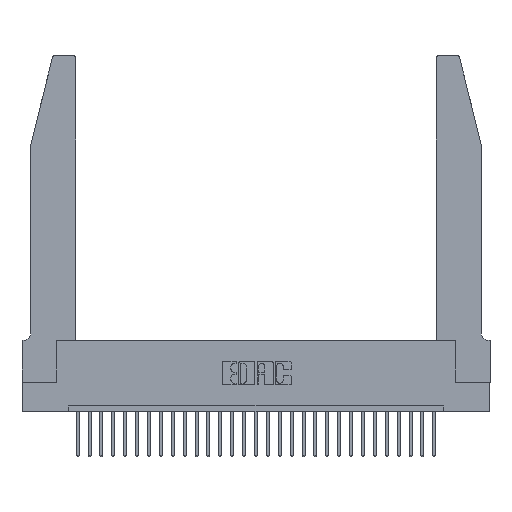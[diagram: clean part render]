
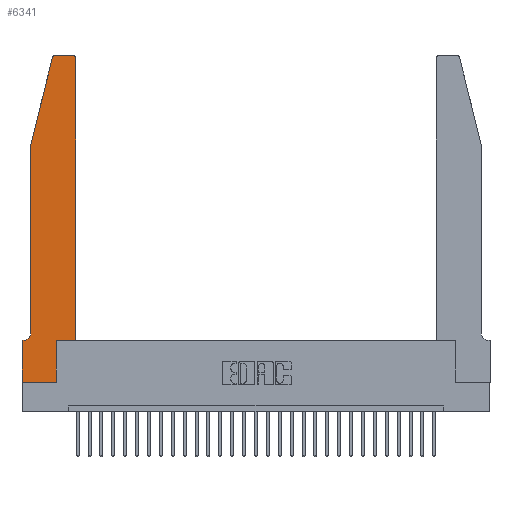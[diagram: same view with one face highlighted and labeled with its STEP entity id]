
A CAD part, top view. The second image highlights one B-rep face of the part: STEP entity #6341.
In plain terms, the highlighted planar face has unit normal (0, 0, 1).
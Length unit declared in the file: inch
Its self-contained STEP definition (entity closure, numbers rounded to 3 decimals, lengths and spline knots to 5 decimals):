
#595 = ORIENTED_EDGE ( 'NONE', *, *, #10351, .T. ) ;
#735 = ORIENTED_EDGE ( 'NONE', *, *, #6248, .T. ) ;
#934 = CARTESIAN_POINT ( 'NONE',  ( 0.0755, 0.35, 0.37 ) ) ;
#1357 = CARTESIAN_POINT ( 'NONE',  ( 0.25487, 2.72718, 0.37 ) ) ;
#1361 = ORIENTED_EDGE ( 'NONE', *, *, #3105, .T. ) ;
#1368 = EDGE_CURVE ( 'NONE', #23495, #5589, #11917, .T. ) ;
#1647 = CARTESIAN_POINT ( 'NONE',  ( 0., 0., 0.37 ) ) ;
#1917 = CARTESIAN_POINT ( 'NONE',  ( 0., 0., 0.37 ) ) ;
#2184 = ORIENTED_EDGE ( 'NONE', *, *, #26930, .T. ) ;
#2777 = CARTESIAN_POINT ( 'NONE',  ( 0.284, 2.72, 0.37 ) ) ;
#3105 = EDGE_CURVE ( 'NONE', #5589, #27038, #28987, .T. ) ;
#3804 = ORIENTED_EDGE ( 'NONE', *, *, #10333, .T. ) ;
#4568 = LINE ( 'NONE', #23553, #22810 ) ;
#4655 = CARTESIAN_POINT ( 'NONE',  ( 0.4505, 2.72, 0.37 ) ) ;
#4871 = VECTOR ( 'NONE', #26889, 39.37008 ) ;
#5257 = DIRECTION ( 'NONE',  ( 1., 0., 0. ) ) ;
#5456 = VERTEX_POINT ( 'NONE', #12390 ) ;
#5538 = DIRECTION ( 'NONE',  ( 0., 0., 1. ) ) ;
#5582 = CARTESIAN_POINT ( 'NONE',  ( 0.4505, 0.35, 0.37 ) ) ;
#5589 = VERTEX_POINT ( 'NONE', #27062 ) ;
#5603 = CIRCLE ( 'NONE', #28154, 0.07 ) ;
#5796 = LINE ( 'NONE', #25806, #15432 ) ;
#5948 = EDGE_CURVE ( 'NONE', #5456, #9611, #22768, .T. ) ;
#6243 = VERTEX_POINT ( 'NONE', #16514 ) ;
#6248 = EDGE_CURVE ( 'NONE', #14806, #23495, #5603, .T. ) ;
#6341 = ADVANCED_FACE ( 'NONE', ( #29182 ), #28057, .T. ) ;
#6641 = LINE ( 'NONE', #22114, #19127 ) ;
#7485 = ORIENTED_EDGE ( 'NONE', *, *, #12717, .T. ) ;
#7992 = CIRCLE ( 'NONE', #11518, 0.03 ) ;
#9493 = LINE ( 'NONE', #1917, #4871 ) ;
#9611 = VERTEX_POINT ( 'NONE', #21404 ) ;
#9861 = VECTOR ( 'NONE', #11960, 39.37008 ) ;
#9874 = ORIENTED_EDGE ( 'NONE', *, *, #5948, .T. ) ;
#10333 = EDGE_CURVE ( 'NONE', #9611, #28482, #19593, .T. ) ;
#10351 = EDGE_CURVE ( 'NONE', #28482, #28876, #4568, .T. ) ;
#10676 = DIRECTION ( 'NONE',  ( 0., -1., 0. ) ) ;
#11081 = CARTESIAN_POINT ( 'NONE',  ( 0.2865, 0., 0.37 ) ) ;
#11518 = AXIS2_PLACEMENT_3D ( 'NONE', #19491, #15108, #14905 ) ;
#11917 = LINE ( 'NONE', #934, #17292 ) ;
#11960 = DIRECTION ( 'NONE',  ( -1., 0., 0. ) ) ;
#12302 = CARTESIAN_POINT ( 'NONE',  ( 0.0055, 0.42, 0.37 ) ) ;
#12317 = VERTEX_POINT ( 'NONE', #5582 ) ;
#12390 = CARTESIAN_POINT ( 'NONE',  ( 0.4205, 2.75, 0.37 ) ) ;
#12717 = EDGE_CURVE ( 'NONE', #25832, #5456, #7992, .T. ) ;
#13031 = EDGE_CURVE ( 'NONE', #24808, #6243, #18321, .T. ) ;
#13212 = AXIS2_PLACEMENT_3D ( 'NONE', #18994, #5538, #14721 ) ;
#13441 = CARTESIAN_POINT ( 'NONE',  ( 0.4505, 0.35, 0.37 ) ) ;
#13883 = CARTESIAN_POINT ( 'NONE',  ( 0., 0., 0.37 ) ) ;
#14362 = DIRECTION ( 'NONE',  ( 0., 0., 1. ) ) ;
#14420 = LINE ( 'NONE', #13441, #28045 ) ;
#14721 = DIRECTION ( 'NONE',  ( 1., 0., 0. ) ) ;
#14806 = VERTEX_POINT ( 'NONE', #28997 ) ;
#14905 = DIRECTION ( 'NONE',  ( 1., 0., 0. ) ) ;
#15108 = DIRECTION ( 'NONE',  ( 0., 0., 1. ) ) ;
#15432 = VECTOR ( 'NONE', #25898, 39.37008 ) ;
#16514 = CARTESIAN_POINT ( 'NONE',  ( 0.2865, 0.35, 0.37 ) ) ;
#16920 = DIRECTION ( 'NONE',  ( -0.239, -0.971, 0. ) ) ;
#17146 = VECTOR ( 'NONE', #10676, 39.37008 ) ;
#17292 = VECTOR ( 'NONE', #23721, 39.37008 ) ;
#18321 = LINE ( 'NONE', #21827, #26249 ) ;
#18994 = CARTESIAN_POINT ( 'NONE',  ( 0., 0.35, 0.37 ) ) ;
#19101 = DIRECTION ( 'NONE',  ( 0., 0., -1. ) ) ;
#19127 = VECTOR ( 'NONE', #26721, 39.37008 ) ;
#19491 = CARTESIAN_POINT ( 'NONE',  ( 0.4205, 2.72, 0.37 ) ) ;
#19593 = CIRCLE ( 'NONE', #24201, 0.03 ) ;
#20151 = ORIENTED_EDGE ( 'NONE', *, *, #25614, .T. ) ;
#20570 = ORIENTED_EDGE ( 'NONE', *, *, #28171, .T. ) ;
#21404 = CARTESIAN_POINT ( 'NONE',  ( 0.284, 2.75, 0.37 ) ) ;
#21416 = DIRECTION ( 'NONE',  ( -1., 0., 0. ) ) ;
#21457 = ORIENTED_EDGE ( 'NONE', *, *, #28980, .T. ) ;
#21548 = CARTESIAN_POINT ( 'NONE',  ( 0.0055, 0.35, 0.37 ) ) ;
#21827 = CARTESIAN_POINT ( 'NONE',  ( 0.2865, 0.35, 0.37 ) ) ;
#22114 = CARTESIAN_POINT ( 'NONE',  ( 0.4505, 0.35, 0.37 ) ) ;
#22639 = DIRECTION ( 'NONE',  ( 0., 1., 0. ) ) ;
#22768 = LINE ( 'NONE', #27805, #9861 ) ;
#22810 = VECTOR ( 'NONE', #16920, 39.37008 ) ;
#23495 = VERTEX_POINT ( 'NONE', #21548 ) ;
#23553 = CARTESIAN_POINT ( 'NONE',  ( 0.0755, 2., 0.37 ) ) ;
#23721 = DIRECTION ( 'NONE',  ( -1., 0., 0. ) ) ;
#24201 = AXIS2_PLACEMENT_3D ( 'NONE', #2777, #14362, #5257 ) ;
#24554 = ORIENTED_EDGE ( 'NONE', *, *, #1368, .T. ) ;
#24808 = VERTEX_POINT ( 'NONE', #11081 ) ;
#25614 = EDGE_CURVE ( 'NONE', #27038, #24808, #9493, .T. ) ;
#25806 = CARTESIAN_POINT ( 'NONE',  ( 0.0755, 2., 0.37 ) ) ;
#25832 = VERTEX_POINT ( 'NONE', #4655 ) ;
#25898 = DIRECTION ( 'NONE',  ( 0., -1., 0. ) ) ;
#26249 = VECTOR ( 'NONE', #26432, 39.37008 ) ;
#26432 = DIRECTION ( 'NONE',  ( 0., 1., 0. ) ) ;
#26721 = DIRECTION ( 'NONE',  ( 1., 0., 0. ) ) ;
#26889 = DIRECTION ( 'NONE',  ( 1., 0., 0. ) ) ;
#26930 = EDGE_CURVE ( 'NONE', #6243, #12317, #6641, .T. ) ;
#27038 = VERTEX_POINT ( 'NONE', #13883 ) ;
#27062 = CARTESIAN_POINT ( 'NONE',  ( 0., 0.35, 0.37 ) ) ;
#27420 = CARTESIAN_POINT ( 'NONE',  ( 0.0755, 2., 0.37 ) ) ;
#27805 = CARTESIAN_POINT ( 'NONE',  ( 0.2605, 2.75, 0.37 ) ) ;
#28045 = VECTOR ( 'NONE', #22639, 39.37008 ) ;
#28057 = PLANE ( 'NONE',  #13212 ) ;
#28154 = AXIS2_PLACEMENT_3D ( 'NONE', #12302, #19101, #21416 ) ;
#28171 = EDGE_CURVE ( 'NONE', #12317, #25832, #14420, .T. ) ;
#28449 = ORIENTED_EDGE ( 'NONE', *, *, #13031, .T. ) ;
#28482 = VERTEX_POINT ( 'NONE', #1357 ) ;
#28876 = VERTEX_POINT ( 'NONE', #27420 ) ;
#28980 = EDGE_CURVE ( 'NONE', #28876, #14806, #5796, .T. ) ;
#28987 = LINE ( 'NONE', #1647, #17146 ) ;
#28997 = CARTESIAN_POINT ( 'NONE',  ( 0.0755, 0.42, 0.37 ) ) ;
#29182 = FACE_OUTER_BOUND ( 'NONE', #29474, .T. ) ;
#29474 = EDGE_LOOP ( 'NONE', ( #9874, #3804, #595, #21457, #735, #24554, #1361, #20151, #28449, #2184, #20570, #7485 ) ) ;
